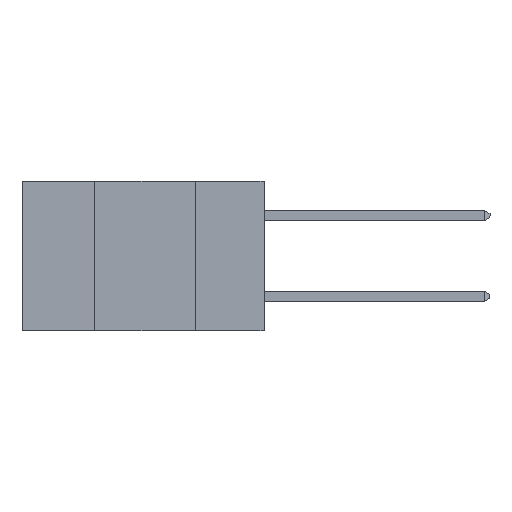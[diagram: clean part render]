
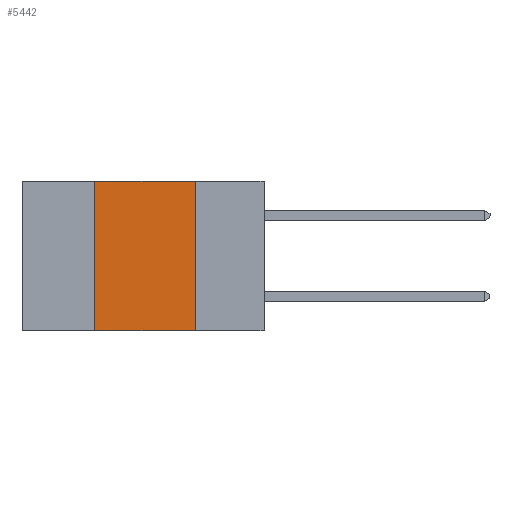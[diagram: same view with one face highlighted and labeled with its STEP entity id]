
A CAD part, left-side view. The second image highlights one B-rep face of the part: STEP entity #5442.
In plain terms, the highlighted planar face has unit normal (-1, 0, 0).
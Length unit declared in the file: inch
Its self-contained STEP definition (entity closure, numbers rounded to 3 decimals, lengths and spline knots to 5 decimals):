
#751 = CARTESIAN_POINT ( 'NONE',  ( 0., 0.17, 0. ) ) ;
#1213 = ORIENTED_EDGE ( 'NONE', *, *, #5581, .F. ) ;
#1490 = DIRECTION ( 'NONE',  ( 0., -1., 0. ) ) ;
#1620 = CARTESIAN_POINT ( 'NONE',  ( 0., 0.42, -0.37 ) ) ;
#1712 = ORIENTED_EDGE ( 'NONE', *, *, #4253, .T. ) ;
#2178 = LINE ( 'NONE', #13190, #13510 ) ;
#3128 = VERTEX_POINT ( 'NONE', #1620 ) ;
#4232 = EDGE_LOOP ( 'NONE', ( #13082, #1213, #5468, #1712 ) ) ;
#4253 = EDGE_CURVE ( 'NONE', #3128, #8166, #12118, .T. ) ;
#4312 = DIRECTION ( 'NONE',  ( 0., 0., -1. ) ) ;
#5310 = EDGE_CURVE ( 'NONE', #3128, #6252, #2178, .T. ) ;
#5442 = ADVANCED_FACE ( 'NONE', ( #18184 ), #14991, .F. ) ;
#5468 = ORIENTED_EDGE ( 'NONE', *, *, #5310, .F. ) ;
#5581 = EDGE_CURVE ( 'NONE', #6252, #16066, #19794, .T. ) ;
#5639 = AXIS2_PLACEMENT_3D ( 'NONE', #6779, #13952, #10998 ) ;
#6252 = VERTEX_POINT ( 'NONE', #16790 ) ;
#6344 = EDGE_CURVE ( 'NONE', #16066, #8166, #9676, .T. ) ;
#6779 = CARTESIAN_POINT ( 'NONE',  ( 0., 0.6, 0. ) ) ;
#8166 = VERTEX_POINT ( 'NONE', #19721 ) ;
#8323 = VECTOR ( 'NONE', #1490, 39.37008 ) ;
#8576 = VECTOR ( 'NONE', #17527, 39.37008 ) ;
#9676 = LINE ( 'NONE', #10826, #17675 ) ;
#10826 = CARTESIAN_POINT ( 'NONE',  ( 0., 0.17, 0. ) ) ;
#10998 = DIRECTION ( 'NONE',  ( 0., 0., -1. ) ) ;
#12118 = LINE ( 'NONE', #15157, #8576 ) ;
#13082 = ORIENTED_EDGE ( 'NONE', *, *, #6344, .F. ) ;
#13190 = CARTESIAN_POINT ( 'NONE',  ( 0., 0.42, 0. ) ) ;
#13510 = VECTOR ( 'NONE', #15142, 39.37008 ) ;
#13952 = DIRECTION ( 'NONE',  ( 1., 0., 0. ) ) ;
#14991 = PLANE ( 'NONE',  #5639 ) ;
#15142 = DIRECTION ( 'NONE',  ( 0., 0., 1. ) ) ;
#15157 = CARTESIAN_POINT ( 'NONE',  ( 0., 0.6, -0.37 ) ) ;
#16066 = VERTEX_POINT ( 'NONE', #751 ) ;
#16790 = CARTESIAN_POINT ( 'NONE',  ( 0., 0.42, 0. ) ) ;
#17231 = CARTESIAN_POINT ( 'NONE',  ( 0., 0.6, 0. ) ) ;
#17527 = DIRECTION ( 'NONE',  ( 0., -1., 0. ) ) ;
#17675 = VECTOR ( 'NONE', #4312, 39.37008 ) ;
#18184 = FACE_OUTER_BOUND ( 'NONE', #4232, .T. ) ;
#19721 = CARTESIAN_POINT ( 'NONE',  ( 0., 0.17, -0.37 ) ) ;
#19794 = LINE ( 'NONE', #17231, #8323 ) ;
